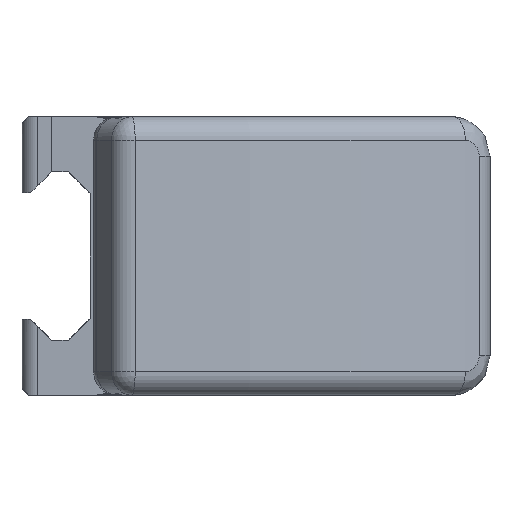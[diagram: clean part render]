
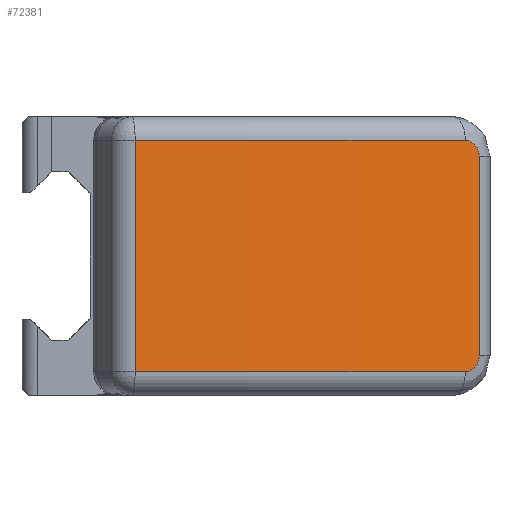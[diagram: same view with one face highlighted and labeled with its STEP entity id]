
A CAD part, left-side view. The second image highlights one B-rep face of the part: STEP entity #72381.
In plain terms, the highlighted cylindrical face has radius 107.63 mm (diameter 215.261 mm), a partial arc.
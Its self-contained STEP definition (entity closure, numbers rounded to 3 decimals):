
#41=B_SPLINE_CURVE_WITH_KNOTS('',3,(#108484,#108485,#108486,#108487,#108488,
#108489),.UNSPECIFIED.,.F.,.F.,(4,1,1,4),(0.,0.09,0.18,
0.314),.UNSPECIFIED.);
#53=B_SPLINE_CURVE_WITH_KNOTS('',3,(#117450,#117451,#117452,#117453,#117454,
#117455),.UNSPECIFIED.,.F.,.F.,(4,1,1,4),(0.,0.09,0.18,
0.314),.UNSPECIFIED.);
#171=CIRCLE('',#75401,107.631);
#185=CIRCLE('',#78175,107.631);
#215=CYLINDRICAL_SURFACE('',#78174,107.631);
#5767=FACE_OUTER_BOUND('',#11444,.T.);
#11444=EDGE_LOOP('',(#60078,#60079,#60080,#60081,#60082,#60083));
#20524=LINE('',#117440,#29630);
#20527=LINE('',#117448,#29633);
#29630=VECTOR('',#98572,10.);
#29633=VECTOR('',#98581,10.);
#31648=VERTEX_POINT('',#108439);
#31650=VERTEX_POINT('',#108449);
#31651=VERTEX_POINT('',#108482);
#33323=VERTEX_POINT('',#117439);
#33325=VERTEX_POINT('',#117447);
#33326=VERTEX_POINT('',#117449);
#38030=EDGE_CURVE('',#31648,#31650,#171,.T.);
#38032=EDGE_CURVE('',#31650,#31651,#41,.T.);
#42462=EDGE_CURVE('',#33323,#31648,#20524,.T.);
#42466=EDGE_CURVE('',#31651,#33325,#20527,.T.);
#42467=EDGE_CURVE('',#33326,#33325,#53,.T.);
#42468=EDGE_CURVE('',#33323,#33326,#185,.T.);
#60078=ORIENTED_EDGE('',*,*,#42466,.T.);
#60079=ORIENTED_EDGE('',*,*,#42467,.F.);
#60080=ORIENTED_EDGE('',*,*,#42468,.F.);
#60081=ORIENTED_EDGE('',*,*,#42462,.T.);
#60082=ORIENTED_EDGE('',*,*,#38030,.T.);
#60083=ORIENTED_EDGE('',*,*,#38032,.T.);
#72381=ADVANCED_FACE('',(#5767),#215,.T.);
#75401=AXIS2_PLACEMENT_3D('',#108451,#88631,#88632);
#78174=AXIS2_PLACEMENT_3D('',#117446,#98579,#98580);
#78175=AXIS2_PLACEMENT_3D('',#117456,#98582,#98583);
#88631=DIRECTION('center_axis',(0.,0.,
1.));
#88632=DIRECTION('ref_axis',(-0.942,-0.334,0.));
#98572=DIRECTION('',(0.,0.,-1.));
#98579=DIRECTION('center_axis',(0.,0.,
-1.));
#98580=DIRECTION('ref_axis',(-0.993,-0.114,0.));
#98581=DIRECTION('',(0.,0.,1.));
#98582=DIRECTION('center_axis',(0.,0.,
1.));
#98583=DIRECTION('ref_axis',(-0.942,-0.334,0.));
#108439=CARTESIAN_POINT('',(-110.965,-45.368,-10.958));
#108449=CARTESIAN_POINT('',(-96.064,-87.31,-10.958));
#108451=CARTESIAN_POINT('Origin',(-4.286,-31.086,-10.958));
#108482=CARTESIAN_POINT('',(-94.972,-89.055,-8.958));
#108484=CARTESIAN_POINT('Ctrl Pts',(-96.064,-87.31,
-10.958));
#108485=CARTESIAN_POINT('Ctrl Pts',(-95.903,-87.573,-10.958));
#108486=CARTESIAN_POINT('Ctrl Pts',(-95.58,-88.095,
-10.821));
#108487=CARTESIAN_POINT('Ctrl Pts',(-95.118,-88.828,
-10.152));
#108488=CARTESIAN_POINT('Ctrl Pts',(-94.972,-89.055,
-9.406));
#108489=CARTESIAN_POINT('Ctrl Pts',(-94.972,-89.055,
-8.958));
#117439=CARTESIAN_POINT('',(-110.965,-45.368,18.413));
#117440=CARTESIAN_POINT('',(-110.965,-45.368,-13.958));
#117446=CARTESIAN_POINT('Origin',(-4.286,-31.086,21.413));
#117447=CARTESIAN_POINT('',(-94.972,-89.055,16.413));
#117448=CARTESIAN_POINT('',(-94.972,-89.055,-13.958));
#117449=CARTESIAN_POINT('',(-96.064,-87.31,18.413));
#117450=CARTESIAN_POINT('Ctrl Pts',(-96.064,-87.31,
18.413));
#117451=CARTESIAN_POINT('Ctrl Pts',(-95.903,-87.573,18.413));
#117452=CARTESIAN_POINT('Ctrl Pts',(-95.58,-88.095,
18.276));
#117453=CARTESIAN_POINT('Ctrl Pts',(-95.118,-88.828,
17.607));
#117454=CARTESIAN_POINT('Ctrl Pts',(-94.972,-89.055,
16.862));
#117455=CARTESIAN_POINT('Ctrl Pts',(-94.972,-89.055,
16.413));
#117456=CARTESIAN_POINT('Origin',(-4.286,-31.086,18.413));
